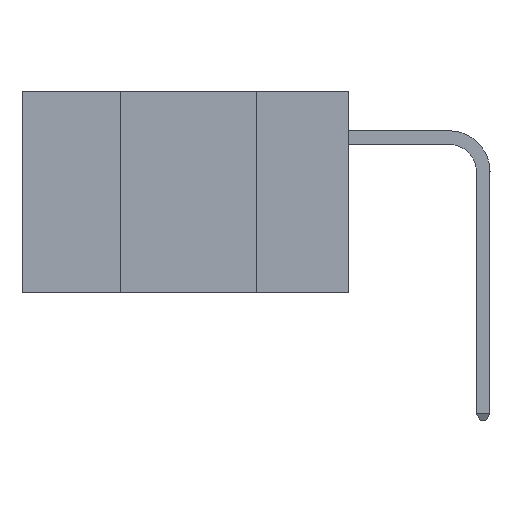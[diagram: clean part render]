
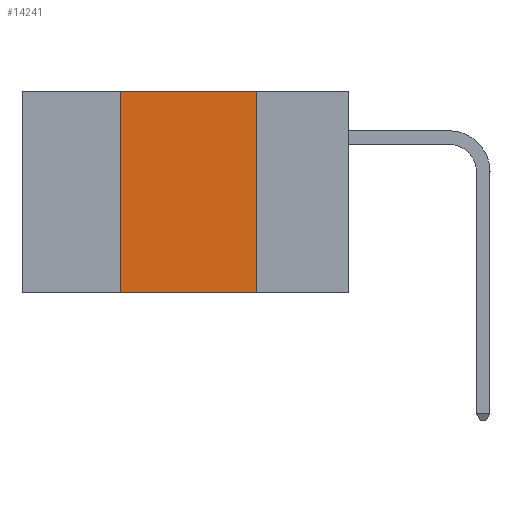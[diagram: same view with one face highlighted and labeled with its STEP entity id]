
A CAD part, left-side view. The second image highlights one B-rep face of the part: STEP entity #14241.
In plain terms, the highlighted planar face has unit normal (-1, 0, 0).
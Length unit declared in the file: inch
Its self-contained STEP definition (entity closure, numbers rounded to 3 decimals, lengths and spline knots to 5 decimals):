
#482 = AXIS2_PLACEMENT_3D ( 'NONE', #13721, #3736, #17796 ) ;
#1082 = LINE ( 'NONE', #25985, #6473 ) ;
#1897 = VERTEX_POINT ( 'NONE', #13685 ) ;
#3396 = DIRECTION ( 'NONE',  ( 0., -1., 0. ) ) ;
#3736 = DIRECTION ( 'NONE',  ( 1., 0., 0. ) ) ;
#3737 = VECTOR ( 'NONE', #15874, 39.37008 ) ;
#3849 = DIRECTION ( 'NONE',  ( 0., -1., 0. ) ) ;
#4584 = EDGE_CURVE ( 'NONE', #18267, #1897, #13839, .T. ) ;
#4622 = ORIENTED_EDGE ( 'NONE', *, *, #4584, .T. ) ;
#5942 = EDGE_CURVE ( 'NONE', #18267, #20761, #15002, .T. ) ;
#6105 = EDGE_LOOP ( 'NONE', ( #24481, #20064, #21491, #4622 ) ) ;
#6473 = VECTOR ( 'NONE', #3849, 39.37008 ) ;
#7060 = LINE ( 'NONE', #20417, #7695 ) ;
#7695 = VECTOR ( 'NONE', #18361, 39.37008 ) ;
#7710 = PLANE ( 'NONE',  #482 ) ;
#7750 = CARTESIAN_POINT ( 'NONE',  ( 0., 0.42, 0. ) ) ;
#8620 = EDGE_CURVE ( 'NONE', #21003, #1897, #7060, .T. ) ;
#9449 = CARTESIAN_POINT ( 'NONE',  ( 0., 0.6, -0.37 ) ) ;
#11363 = EDGE_CURVE ( 'NONE', #20761, #21003, #1082, .T. ) ;
#12296 = FACE_OUTER_BOUND ( 'NONE', #6105, .T. ) ;
#13685 = CARTESIAN_POINT ( 'NONE',  ( 0., 0.17, -0.37 ) ) ;
#13721 = CARTESIAN_POINT ( 'NONE',  ( 0., 0.6, 0. ) ) ;
#13839 = LINE ( 'NONE', #9449, #24656 ) ;
#14241 = ADVANCED_FACE ( 'NONE', ( #12296 ), #7710, .F. ) ;
#14435 = CARTESIAN_POINT ( 'NONE',  ( 0., 0.17, 0. ) ) ;
#15002 = LINE ( 'NONE', #19923, #3737 ) ;
#15874 = DIRECTION ( 'NONE',  ( 0., 0., 1. ) ) ;
#17796 = DIRECTION ( 'NONE',  ( 0., 0., -1. ) ) ;
#18267 = VERTEX_POINT ( 'NONE', #20550 ) ;
#18361 = DIRECTION ( 'NONE',  ( 0., 0., -1. ) ) ;
#19923 = CARTESIAN_POINT ( 'NONE',  ( 0., 0.42, 0. ) ) ;
#20064 = ORIENTED_EDGE ( 'NONE', *, *, #11363, .F. ) ;
#20417 = CARTESIAN_POINT ( 'NONE',  ( 0., 0.17, 0. ) ) ;
#20550 = CARTESIAN_POINT ( 'NONE',  ( 0., 0.42, -0.37 ) ) ;
#20761 = VERTEX_POINT ( 'NONE', #7750 ) ;
#21003 = VERTEX_POINT ( 'NONE', #14435 ) ;
#21491 = ORIENTED_EDGE ( 'NONE', *, *, #5942, .F. ) ;
#24481 = ORIENTED_EDGE ( 'NONE', *, *, #8620, .F. ) ;
#24656 = VECTOR ( 'NONE', #3396, 39.37008 ) ;
#25985 = CARTESIAN_POINT ( 'NONE',  ( 0., 0.6, 0. ) ) ;
